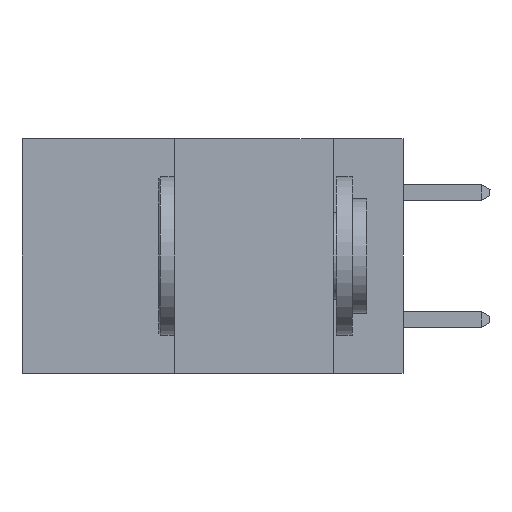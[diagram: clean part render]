
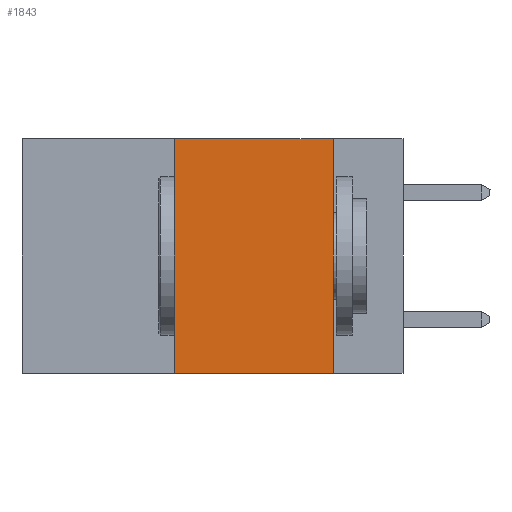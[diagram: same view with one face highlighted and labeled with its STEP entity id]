
A CAD part, left-side view. The second image highlights one B-rep face of the part: STEP entity #1843.
In plain terms, the highlighted planar face has unit normal (-1, 0, 0).
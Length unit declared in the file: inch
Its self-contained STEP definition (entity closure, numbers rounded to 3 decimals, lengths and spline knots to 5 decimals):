
#290 = ORIENTED_EDGE ( 'NONE', *, *, #9391, .F. ) ;
#324 = DIRECTION ( 'NONE',  ( 0., -1., 0. ) ) ;
#1211 = DIRECTION ( 'NONE',  ( 0., 0., 1. ) ) ;
#1348 = EDGE_CURVE ( 'NONE', #13037, #8630, #17229, .T. ) ;
#1843 = ADVANCED_FACE ( 'NONE', ( #23494 ), #8642, .F. ) ;
#2977 = VECTOR ( 'NONE', #324, 39.37008 ) ;
#4157 = LINE ( 'NONE', #8145, #2977 ) ;
#4227 = VECTOR ( 'NONE', #5524, 39.37008 ) ;
#4854 = LINE ( 'NONE', #24512, #4227 ) ;
#4917 = CARTESIAN_POINT ( 'NONE',  ( 0., 0.6, 0. ) ) ;
#5524 = DIRECTION ( 'NONE',  ( 0., -1., 0. ) ) ;
#7580 = CARTESIAN_POINT ( 'NONE',  ( 0., 0.36, -0.37 ) ) ;
#8145 = CARTESIAN_POINT ( 'NONE',  ( 0., 0.6, -0.37 ) ) ;
#8630 = VERTEX_POINT ( 'NONE', #9230 ) ;
#8642 = PLANE ( 'NONE',  #20450 ) ;
#8804 = EDGE_LOOP ( 'NONE', ( #21405, #290, #22520, #19141 ) ) ;
#9230 = CARTESIAN_POINT ( 'NONE',  ( 0., 0.36, 0. ) ) ;
#9391 = EDGE_CURVE ( 'NONE', #8630, #17313, #4854, .T. ) ;
#13037 = VERTEX_POINT ( 'NONE', #7580 ) ;
#14120 = VECTOR ( 'NONE', #18534, 39.37008 ) ;
#14253 = VECTOR ( 'NONE', #1211, 39.37008 ) ;
#16535 = EDGE_CURVE ( 'NONE', #17313, #19121, #17718, .T. ) ;
#16586 = CARTESIAN_POINT ( 'NONE',  ( 0., 0.11, 0. ) ) ;
#17005 = DIRECTION ( 'NONE',  ( 0., 0., -1. ) ) ;
#17229 = LINE ( 'NONE', #20130, #14253 ) ;
#17313 = VERTEX_POINT ( 'NONE', #21034 ) ;
#17718 = LINE ( 'NONE', #16586, #14120 ) ;
#18534 = DIRECTION ( 'NONE',  ( 0., 0., -1. ) ) ;
#19121 = VERTEX_POINT ( 'NONE', #24382 ) ;
#19141 = ORIENTED_EDGE ( 'NONE', *, *, #19599, .T. ) ;
#19599 = EDGE_CURVE ( 'NONE', #13037, #19121, #4157, .T. ) ;
#20130 = CARTESIAN_POINT ( 'NONE',  ( 0., 0.36, 0. ) ) ;
#20450 = AXIS2_PLACEMENT_3D ( 'NONE', #4917, #23982, #17005 ) ;
#21034 = CARTESIAN_POINT ( 'NONE',  ( 0., 0.11, 0. ) ) ;
#21405 = ORIENTED_EDGE ( 'NONE', *, *, #16535, .F. ) ;
#22520 = ORIENTED_EDGE ( 'NONE', *, *, #1348, .F. ) ;
#23494 = FACE_OUTER_BOUND ( 'NONE', #8804, .T. ) ;
#23982 = DIRECTION ( 'NONE',  ( 1., 0., 0. ) ) ;
#24382 = CARTESIAN_POINT ( 'NONE',  ( 0., 0.11, -0.37 ) ) ;
#24512 = CARTESIAN_POINT ( 'NONE',  ( 0., 0.6, 0. ) ) ;
